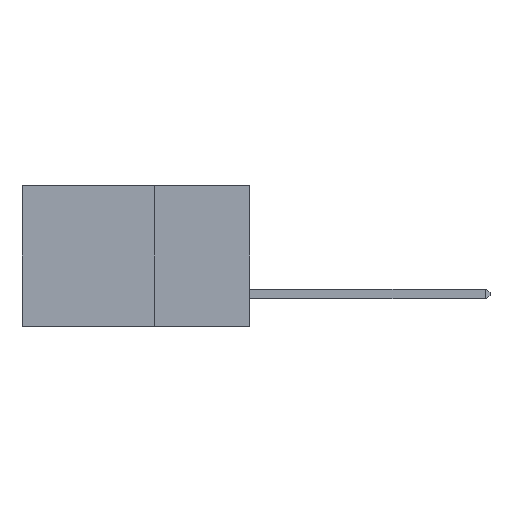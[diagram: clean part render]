
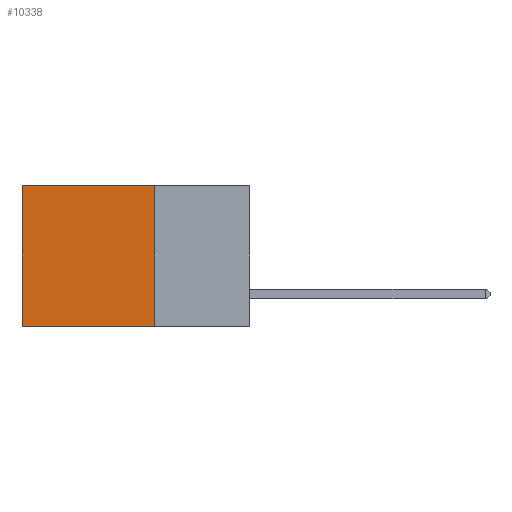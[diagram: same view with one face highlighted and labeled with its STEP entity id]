
A CAD part, left-side view. The second image highlights one B-rep face of the part: STEP entity #10338.
In plain terms, the highlighted planar face has unit normal (-1, 0, 0).
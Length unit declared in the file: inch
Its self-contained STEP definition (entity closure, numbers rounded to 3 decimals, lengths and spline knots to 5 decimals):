
#365 = EDGE_CURVE ( 'NONE', #19822, #16875, #18917, .T. ) ;
#1057 = EDGE_CURVE ( 'NONE', #6291, #19822, #1873, .T. ) ;
#1081 = CARTESIAN_POINT ( 'NONE',  ( 0.2875, 0.25, 0. ) ) ;
#1294 = VECTOR ( 'NONE', #2902, 39.37008 ) ;
#1488 = VECTOR ( 'NONE', #20343, 39.37008 ) ;
#1873 = LINE ( 'NONE', #1081, #1294 ) ;
#2902 = DIRECTION ( 'NONE',  ( 0., 1., 0. ) ) ;
#3876 = CARTESIAN_POINT ( 'NONE',  ( 0.2875, 0.25, -0.37 ) ) ;
#4680 = CARTESIAN_POINT ( 'NONE',  ( 0.2875, 0.6, 0. ) ) ;
#5443 = EDGE_CURVE ( 'NONE', #6291, #21758, #20169, .T. ) ;
#5544 = ORIENTED_EDGE ( 'NONE', *, *, #7009, .F. ) ;
#5622 = ORIENTED_EDGE ( 'NONE', *, *, #1057, .T. ) ;
#5854 = CARTESIAN_POINT ( 'NONE',  ( 0.2875, 0.25, 0. ) ) ;
#6291 = VERTEX_POINT ( 'NONE', #10053 ) ;
#7009 = EDGE_CURVE ( 'NONE', #21758, #16875, #19842, .T. ) ;
#8288 = CARTESIAN_POINT ( 'NONE',  ( 0.2875, 0.6, -0.37 ) ) ;
#8316 = ORIENTED_EDGE ( 'NONE', *, *, #365, .T. ) ;
#9014 = AXIS2_PLACEMENT_3D ( 'NONE', #10498, #22262, #12219 ) ;
#9412 = DIRECTION ( 'NONE',  ( 0., 0., -1. ) ) ;
#9933 = DIRECTION ( 'NONE',  ( 0., 0., -1. ) ) ;
#10053 = CARTESIAN_POINT ( 'NONE',  ( 0.2875, 0.25, 0. ) ) ;
#10338 = ADVANCED_FACE ( 'NONE', ( #15240 ), #20591, .F. ) ;
#10498 = CARTESIAN_POINT ( 'NONE',  ( 0.2875, 0.25, 0. ) ) ;
#10912 = EDGE_LOOP ( 'NONE', ( #8316, #5544, #18410, #5622 ) ) ;
#11888 = CARTESIAN_POINT ( 'NONE',  ( 0.2875, 0.25, -0.37 ) ) ;
#12219 = DIRECTION ( 'NONE',  ( 0., 0., -1. ) ) ;
#14424 = VECTOR ( 'NONE', #9933, 39.37008 ) ;
#15240 = FACE_OUTER_BOUND ( 'NONE', #10912, .T. ) ;
#15716 = VECTOR ( 'NONE', #9412, 39.37008 ) ;
#16875 = VERTEX_POINT ( 'NONE', #8288 ) ;
#18410 = ORIENTED_EDGE ( 'NONE', *, *, #5443, .F. ) ;
#18917 = LINE ( 'NONE', #4680, #14424 ) ;
#19822 = VERTEX_POINT ( 'NONE', #20954 ) ;
#19842 = LINE ( 'NONE', #11888, #1488 ) ;
#20169 = LINE ( 'NONE', #5854, #15716 ) ;
#20343 = DIRECTION ( 'NONE',  ( 0., 1., 0. ) ) ;
#20591 = PLANE ( 'NONE',  #9014 ) ;
#20954 = CARTESIAN_POINT ( 'NONE',  ( 0.2875, 0.6, 0. ) ) ;
#21758 = VERTEX_POINT ( 'NONE', #3876 ) ;
#22262 = DIRECTION ( 'NONE',  ( 1., 0., 0. ) ) ;
